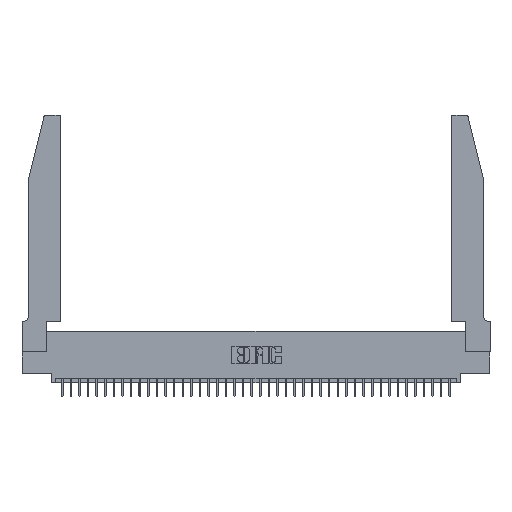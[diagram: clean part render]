
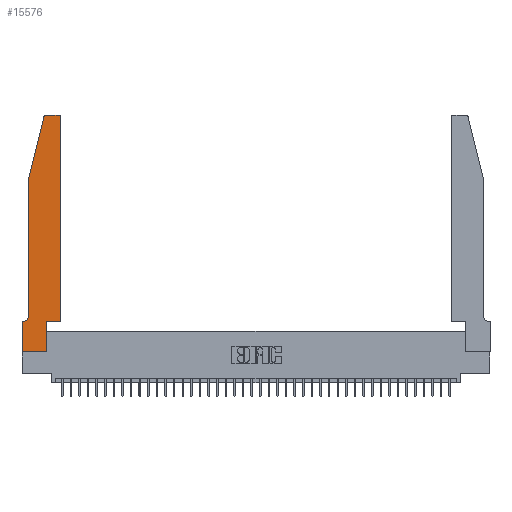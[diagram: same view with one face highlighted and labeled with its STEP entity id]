
A CAD part, top view. The second image highlights one B-rep face of the part: STEP entity #15576.
In plain terms, the highlighted planar face has unit normal (0, 0, 1).
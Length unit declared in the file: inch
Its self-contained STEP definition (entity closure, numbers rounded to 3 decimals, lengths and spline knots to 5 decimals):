
#157 = DIRECTION ( 'NONE',  ( 0., 0., 1. ) ) ;
#402 = VERTEX_POINT ( 'NONE', #11105 ) ;
#771 = VERTEX_POINT ( 'NONE', #9540 ) ;
#1636 = CARTESIAN_POINT ( 'NONE',  ( 0., 0., 0.37 ) ) ;
#1685 = EDGE_CURVE ( 'NONE', #24414, #39513, #15645, .T. ) ;
#2682 = EDGE_CURVE ( 'NONE', #33208, #26452, #38345, .T. ) ;
#2697 = EDGE_CURVE ( 'NONE', #39513, #33208, #28141, .T. ) ;
#3215 = DIRECTION ( 'NONE',  ( -0.239, -0.971, 0. ) ) ;
#3314 = CARTESIAN_POINT ( 'NONE',  ( 0., 0.35, 0.37 ) ) ;
#3449 = VERTEX_POINT ( 'NONE', #12223 ) ;
#4204 = EDGE_CURVE ( 'NONE', #7509, #29525, #13472, .T. ) ;
#4477 = ORIENTED_EDGE ( 'NONE', *, *, #2682, .T. ) ;
#5239 = CARTESIAN_POINT ( 'NONE',  ( 0., 0.35, 0.37 ) ) ;
#5868 = VECTOR ( 'NONE', #13744, 39.37008 ) ;
#6391 = CARTESIAN_POINT ( 'NONE',  ( 0.0755, 2., 0.37 ) ) ;
#6414 = VERTEX_POINT ( 'NONE', #11372 ) ;
#6566 = DIRECTION ( 'NONE',  ( 1., 0., 0. ) ) ;
#6893 = LINE ( 'NONE', #10569, #5868 ) ;
#6996 = ORIENTED_EDGE ( 'NONE', *, *, #2697, .T. ) ;
#7509 = VERTEX_POINT ( 'NONE', #32019 ) ;
#7659 = CARTESIAN_POINT ( 'NONE',  ( 0.284, 2.75, 0.37 ) ) ;
#7932 = VECTOR ( 'NONE', #28828, 39.37008 ) ;
#8246 = DIRECTION ( 'NONE',  ( 1., 0., 0. ) ) ;
#9540 = CARTESIAN_POINT ( 'NONE',  ( 0.0055, 0.35, 0.37 ) ) ;
#9905 = VERTEX_POINT ( 'NONE', #36396 ) ;
#9925 = ORIENTED_EDGE ( 'NONE', *, *, #11946, .T. ) ;
#10569 = CARTESIAN_POINT ( 'NONE',  ( 0.2605, 2.75, 0.37 ) ) ;
#11105 = CARTESIAN_POINT ( 'NONE',  ( 0.4505, 2.72, 0.37 ) ) ;
#11372 = CARTESIAN_POINT ( 'NONE',  ( 0.4505, 0.35, 0.37 ) ) ;
#11640 = VECTOR ( 'NONE', #8246, 39.37008 ) ;
#11946 = EDGE_CURVE ( 'NONE', #29525, #3449, #13633, .T. ) ;
#12223 = CARTESIAN_POINT ( 'NONE',  ( 0.0755, 0.42, 0.37 ) ) ;
#12335 = AXIS2_PLACEMENT_3D ( 'NONE', #36176, #17653, #39319 ) ;
#12845 = PLANE ( 'NONE',  #30214 ) ;
#12970 = CARTESIAN_POINT ( 'NONE',  ( 0.0755, 0.35, 0.37 ) ) ;
#13378 = ORIENTED_EDGE ( 'NONE', *, *, #4204, .T. ) ;
#13472 = LINE ( 'NONE', #25170, #28944 ) ;
#13633 = LINE ( 'NONE', #26576, #36401 ) ;
#13744 = DIRECTION ( 'NONE',  ( -1., 0., 0. ) ) ;
#15361 = ORIENTED_EDGE ( 'NONE', *, *, #32106, .T. ) ;
#15576 = ADVANCED_FACE ( 'NONE', ( #15827 ), #12845, .T. ) ;
#15645 = LINE ( 'NONE', #25925, #38423 ) ;
#15827 = FACE_OUTER_BOUND ( 'NONE', #34689, .T. ) ;
#16730 = DIRECTION ( 'NONE',  ( 0., 1., 0. ) ) ;
#16900 = ORIENTED_EDGE ( 'NONE', *, *, #19587, .T. ) ;
#17087 = DIRECTION ( 'NONE',  ( 0., 0., 1. ) ) ;
#17653 = DIRECTION ( 'NONE',  ( 0., 0., -1. ) ) ;
#18026 = AXIS2_PLACEMENT_3D ( 'NONE', #19137, #157, #22215 ) ;
#18051 = VECTOR ( 'NONE', #16730, 39.37008 ) ;
#18629 = VERTEX_POINT ( 'NONE', #7659 ) ;
#19137 = CARTESIAN_POINT ( 'NONE',  ( 0.284, 2.72, 0.37 ) ) ;
#19587 = EDGE_CURVE ( 'NONE', #26452, #6414, #33732, .T. ) ;
#19694 = EDGE_CURVE ( 'NONE', #402, #9905, #37139, .T. ) ;
#20020 = CARTESIAN_POINT ( 'NONE',  ( 0.2865, 0., 0.37 ) ) ;
#20118 = EDGE_CURVE ( 'NONE', #9905, #18629, #6893, .T. ) ;
#22215 = DIRECTION ( 'NONE',  ( 1., 0., 0. ) ) ;
#23511 = CARTESIAN_POINT ( 'NONE',  ( 0.2865, 0.35, 0.37 ) ) ;
#24225 = AXIS2_PLACEMENT_3D ( 'NONE', #35609, #17087, #38752 ) ;
#24290 = LINE ( 'NONE', #38794, #18051 ) ;
#24414 = VERTEX_POINT ( 'NONE', #5239 ) ;
#25125 = ORIENTED_EDGE ( 'NONE', *, *, #19694, .T. ) ;
#25170 = CARTESIAN_POINT ( 'NONE',  ( 0.0755, 2., 0.37 ) ) ;
#25269 = DIRECTION ( 'NONE',  ( 0., 0., 1. ) ) ;
#25904 = ORIENTED_EDGE ( 'NONE', *, *, #20118, .T. ) ;
#25925 = CARTESIAN_POINT ( 'NONE',  ( 0., 0., 0.37 ) ) ;
#26452 = VERTEX_POINT ( 'NONE', #34698 ) ;
#26576 = CARTESIAN_POINT ( 'NONE',  ( 0.0755, 2., 0.37 ) ) ;
#27393 = CIRCLE ( 'NONE', #12335, 0.07 ) ;
#28141 = LINE ( 'NONE', #1636, #11640 ) ;
#28503 = EDGE_CURVE ( 'NONE', #6414, #402, #24290, .T. ) ;
#28828 = DIRECTION ( 'NONE',  ( 1., 0., 0. ) ) ;
#28944 = VECTOR ( 'NONE', #3215, 39.37008 ) ;
#29480 = ORIENTED_EDGE ( 'NONE', *, *, #28503, .T. ) ;
#29525 = VERTEX_POINT ( 'NONE', #6391 ) ;
#29745 = DIRECTION ( 'NONE',  ( 0., 1., 0. ) ) ;
#30214 = AXIS2_PLACEMENT_3D ( 'NONE', #3314, #25269, #6566 ) ;
#32019 = CARTESIAN_POINT ( 'NONE',  ( 0.25487, 2.72718, 0.37 ) ) ;
#32106 = EDGE_CURVE ( 'NONE', #3449, #771, #27393, .T. ) ;
#32306 = ORIENTED_EDGE ( 'NONE', *, *, #1685, .T. ) ;
#33204 = ORIENTED_EDGE ( 'NONE', *, *, #34986, .T. ) ;
#33208 = VERTEX_POINT ( 'NONE', #20020 ) ;
#33732 = LINE ( 'NONE', #34948, #7932 ) ;
#34614 = DIRECTION ( 'NONE',  ( -1., 0., 0. ) ) ;
#34689 = EDGE_LOOP ( 'NONE', ( #25904, #33204, #13378, #9925, #15361, #38647, #32306, #6996, #4477, #16900, #29480, #25125 ) ) ;
#34698 = CARTESIAN_POINT ( 'NONE',  ( 0.2865, 0.35, 0.37 ) ) ;
#34702 = CARTESIAN_POINT ( 'NONE',  ( 0., 0., 0.37 ) ) ;
#34948 = CARTESIAN_POINT ( 'NONE',  ( 0.4505, 0.35, 0.37 ) ) ;
#34986 = EDGE_CURVE ( 'NONE', #18629, #7509, #39372, .T. ) ;
#35493 = VECTOR ( 'NONE', #34614, 39.37008 ) ;
#35609 = CARTESIAN_POINT ( 'NONE',  ( 0.4205, 2.72, 0.37 ) ) ;
#36176 = CARTESIAN_POINT ( 'NONE',  ( 0.0055, 0.42, 0.37 ) ) ;
#36390 = VECTOR ( 'NONE', #29745, 39.37008 ) ;
#36396 = CARTESIAN_POINT ( 'NONE',  ( 0.4205, 2.75, 0.37 ) ) ;
#36401 = VECTOR ( 'NONE', #38941, 39.37008 ) ;
#36476 = LINE ( 'NONE', #12970, #35493 ) ;
#37139 = CIRCLE ( 'NONE', #24225, 0.03 ) ;
#37545 = EDGE_CURVE ( 'NONE', #771, #24414, #36476, .T. ) ;
#38345 = LINE ( 'NONE', #23511, #36390 ) ;
#38423 = VECTOR ( 'NONE', #38429, 39.37008 ) ;
#38429 = DIRECTION ( 'NONE',  ( 0., -1., 0. ) ) ;
#38647 = ORIENTED_EDGE ( 'NONE', *, *, #37545, .T. ) ;
#38752 = DIRECTION ( 'NONE',  ( 1., 0., 0. ) ) ;
#38794 = CARTESIAN_POINT ( 'NONE',  ( 0.4505, 0.35, 0.37 ) ) ;
#38941 = DIRECTION ( 'NONE',  ( 0., -1., 0. ) ) ;
#39319 = DIRECTION ( 'NONE',  ( -1., 0., 0. ) ) ;
#39372 = CIRCLE ( 'NONE', #18026, 0.03 ) ;
#39513 = VERTEX_POINT ( 'NONE', #34702 ) ;
